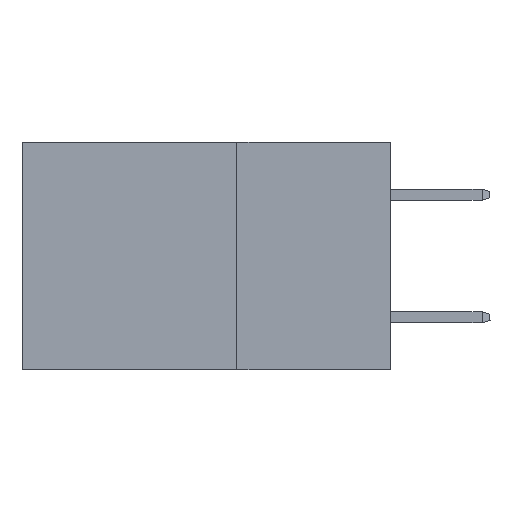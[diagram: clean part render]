
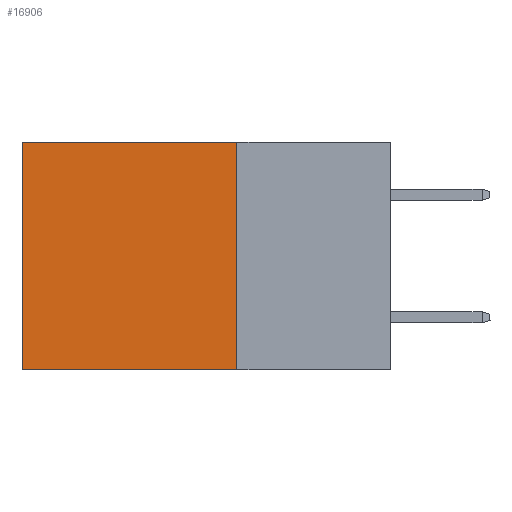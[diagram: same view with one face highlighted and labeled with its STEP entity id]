
A CAD part, left-side view. The second image highlights one B-rep face of the part: STEP entity #16906.
In plain terms, the highlighted planar face has unit normal (-1, 0, 0).
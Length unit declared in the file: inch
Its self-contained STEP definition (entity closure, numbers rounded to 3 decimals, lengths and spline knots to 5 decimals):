
#60 = CARTESIAN_POINT ( 'NONE',  ( 0.2875, 0.6, 0. ) ) ;
#889 = VECTOR ( 'NONE', #7649, 39.37008 ) ;
#1003 = LINE ( 'NONE', #10286, #15471 ) ;
#1570 = DIRECTION ( 'NONE',  ( 0., 1., 0. ) ) ;
#1610 = VERTEX_POINT ( 'NONE', #5338 ) ;
#1762 = EDGE_CURVE ( 'NONE', #5865, #8932, #6980, .T. ) ;
#3520 = DIRECTION ( 'NONE',  ( 0., 0., -1. ) ) ;
#3549 = ORIENTED_EDGE ( 'NONE', *, *, #16971, .F. ) ;
#3905 = EDGE_LOOP ( 'NONE', ( #13097, #4215, #3549, #4988 ) ) ;
#4020 = VECTOR ( 'NONE', #11005, 39.37008 ) ;
#4215 = ORIENTED_EDGE ( 'NONE', *, *, #14455, .F. ) ;
#4242 = CARTESIAN_POINT ( 'NONE',  ( 0.2875, 0.25, 0. ) ) ;
#4492 = CARTESIAN_POINT ( 'NONE',  ( 0.2875, 0.6, 0. ) ) ;
#4988 = ORIENTED_EDGE ( 'NONE', *, *, #1762, .T. ) ;
#5338 = CARTESIAN_POINT ( 'NONE',  ( 0.2875, 0.25, -0.37 ) ) ;
#5544 = EDGE_CURVE ( 'NONE', #8932, #14189, #8591, .T. ) ;
#5737 = CARTESIAN_POINT ( 'NONE',  ( 0.2875, 0.6, -0.37 ) ) ;
#5865 = VERTEX_POINT ( 'NONE', #9903 ) ;
#6247 = DIRECTION ( 'NONE',  ( 1., 0., 0. ) ) ;
#6300 = CARTESIAN_POINT ( 'NONE',  ( 0.2875, 0.25, 0. ) ) ;
#6980 = LINE ( 'NONE', #4242, #7401 ) ;
#7401 = VECTOR ( 'NONE', #1570, 39.37008 ) ;
#7649 = DIRECTION ( 'NONE',  ( 0., 0., -1. ) ) ;
#8591 = LINE ( 'NONE', #60, #4020 ) ;
#8932 = VERTEX_POINT ( 'NONE', #4492 ) ;
#8983 = DIRECTION ( 'NONE',  ( 0., 1., 0. ) ) ;
#9903 = CARTESIAN_POINT ( 'NONE',  ( 0.2875, 0.25, 0. ) ) ;
#10286 = CARTESIAN_POINT ( 'NONE',  ( 0.2875, 0.25, -0.37 ) ) ;
#11005 = DIRECTION ( 'NONE',  ( 0., 0., -1. ) ) ;
#11524 = PLANE ( 'NONE',  #15230 ) ;
#11691 = CARTESIAN_POINT ( 'NONE',  ( 0.2875, 0.25, 0. ) ) ;
#12591 = LINE ( 'NONE', #6300, #889 ) ;
#13097 = ORIENTED_EDGE ( 'NONE', *, *, #5544, .T. ) ;
#14189 = VERTEX_POINT ( 'NONE', #5737 ) ;
#14455 = EDGE_CURVE ( 'NONE', #1610, #14189, #1003, .T. ) ;
#15230 = AXIS2_PLACEMENT_3D ( 'NONE', #11691, #6247, #3520 ) ;
#15471 = VECTOR ( 'NONE', #8983, 39.37008 ) ;
#16789 = FACE_OUTER_BOUND ( 'NONE', #3905, .T. ) ;
#16906 = ADVANCED_FACE ( 'NONE', ( #16789 ), #11524, .F. ) ;
#16971 = EDGE_CURVE ( 'NONE', #5865, #1610, #12591, .T. ) ;
